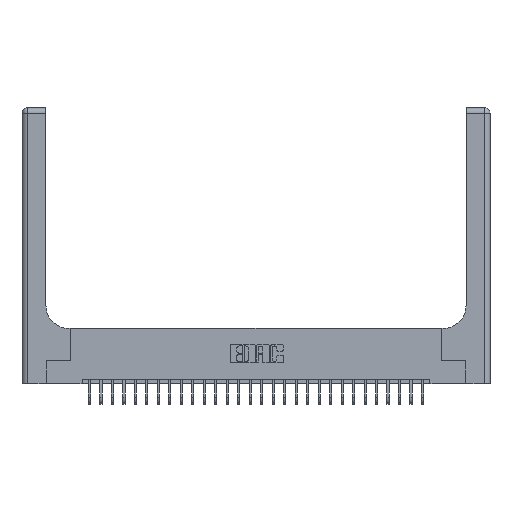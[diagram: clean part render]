
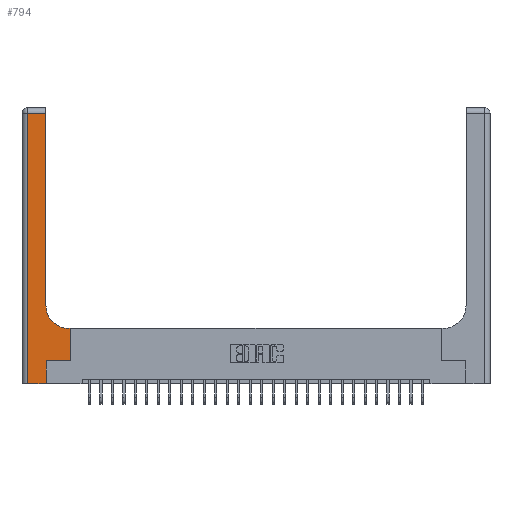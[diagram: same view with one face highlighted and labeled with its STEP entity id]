
A CAD part, top view. The second image highlights one B-rep face of the part: STEP entity #794.
In plain terms, the highlighted planar face has unit normal (0, 0, 1).
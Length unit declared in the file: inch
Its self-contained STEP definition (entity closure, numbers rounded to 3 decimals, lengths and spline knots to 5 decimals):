
#527 = VERTEX_POINT ( 'NONE', #1712 ) ;
#631 = CARTESIAN_POINT ( 'NONE',  ( 0., 2.94, 0.37 ) ) ;
#794 = ADVANCED_FACE ( 'NONE', ( #4896 ), #15321, .F. ) ;
#1518 = ORIENTED_EDGE ( 'NONE', *, *, #18836, .T. ) ;
#1706 = CARTESIAN_POINT ( 'NONE',  ( 0.265, 0.25, 0.37 ) ) ;
#1712 = CARTESIAN_POINT ( 'NONE',  ( 0.528, 0.25, 0.37 ) ) ;
#1751 = CARTESIAN_POINT ( 'NONE',  ( 0.26, 2.94, 0.37 ) ) ;
#1921 = LINE ( 'NONE', #13570, #9097 ) ;
#2032 = ORIENTED_EDGE ( 'NONE', *, *, #19525, .T. ) ;
#2452 = EDGE_CURVE ( 'NONE', #12728, #11250, #26601, .T. ) ;
#3324 = EDGE_CURVE ( 'NONE', #16595, #26419, #27912, .T. ) ;
#3382 = DIRECTION ( 'NONE',  ( 0., 1., 0. ) ) ;
#4296 = DIRECTION ( 'NONE',  ( -1., 0., 0. ) ) ;
#4558 = CARTESIAN_POINT ( 'NONE',  ( 0.06, 2.94, 0.37 ) ) ;
#4566 = CIRCLE ( 'NONE', #7201, 0.25 ) ;
#4896 = FACE_OUTER_BOUND ( 'NONE', #13126, .T. ) ;
#5246 = LINE ( 'NONE', #7978, #27718 ) ;
#5678 = CARTESIAN_POINT ( 'NONE',  ( 0.265, 0., 0.37 ) ) ;
#6216 = CARTESIAN_POINT ( 'NONE',  ( 0.06, 3., 0.37 ) ) ;
#6249 = VECTOR ( 'NONE', #9983, 39.37008 ) ;
#6709 = VERTEX_POINT ( 'NONE', #11661 ) ;
#6754 = VERTEX_POINT ( 'NONE', #14479 ) ;
#7201 = AXIS2_PLACEMENT_3D ( 'NONE', #7893, #12264, #7983 ) ;
#7348 = VECTOR ( 'NONE', #16913, 39.37008 ) ;
#7893 = CARTESIAN_POINT ( 'NONE',  ( 0.51, 0.85, 0.37 ) ) ;
#7978 = CARTESIAN_POINT ( 'NONE',  ( 0.26, 3., 0.37 ) ) ;
#7983 = DIRECTION ( 'NONE',  ( 1., 0., 0. ) ) ;
#8433 = DIRECTION ( 'NONE',  ( 1., 0., 0. ) ) ;
#8619 = CARTESIAN_POINT ( 'NONE',  ( 0., 0., 0.37 ) ) ;
#8766 = CARTESIAN_POINT ( 'NONE',  ( 0., 3., 0.37 ) ) ;
#9097 = VECTOR ( 'NONE', #9546, 39.37008 ) ;
#9546 = DIRECTION ( 'NONE',  ( 0., 1., 0. ) ) ;
#9580 = ORIENTED_EDGE ( 'NONE', *, *, #12456, .T. ) ;
#9902 = ORIENTED_EDGE ( 'NONE', *, *, #3324, .T. ) ;
#9909 = CARTESIAN_POINT ( 'NONE',  ( 0.26, 0.6, 0.37 ) ) ;
#9983 = DIRECTION ( 'NONE',  ( 0., 1., 0. ) ) ;
#10342 = LINE ( 'NONE', #20713, #6249 ) ;
#10442 = EDGE_CURVE ( 'NONE', #22441, #527, #16420, .T. ) ;
#11250 = VERTEX_POINT ( 'NONE', #4558 ) ;
#11661 = CARTESIAN_POINT ( 'NONE',  ( 0.51, 0.6, 0.37 ) ) ;
#12264 = DIRECTION ( 'NONE',  ( 0., 0., -1. ) ) ;
#12456 = EDGE_CURVE ( 'NONE', #11250, #16595, #25415, .T. ) ;
#12728 = VERTEX_POINT ( 'NONE', #1751 ) ;
#13126 = EDGE_LOOP ( 'NONE', ( #2032, #13811, #9580, #9902, #1518, #13508, #14850, #14768, #16028 ) ) ;
#13508 = ORIENTED_EDGE ( 'NONE', *, *, #10442, .T. ) ;
#13570 = CARTESIAN_POINT ( 'NONE',  ( 0.265, 0., 0.37 ) ) ;
#13811 = ORIENTED_EDGE ( 'NONE', *, *, #2452, .T. ) ;
#14378 = EDGE_CURVE ( 'NONE', #527, #17752, #10342, .T. ) ;
#14479 = CARTESIAN_POINT ( 'NONE',  ( 0.26, 0.85, 0.37 ) ) ;
#14768 = ORIENTED_EDGE ( 'NONE', *, *, #17083, .T. ) ;
#14850 = ORIENTED_EDGE ( 'NONE', *, *, #14378, .T. ) ;
#15321 = PLANE ( 'NONE',  #19387 ) ;
#15570 = CARTESIAN_POINT ( 'NONE',  ( 0.06, 0., 0.37 ) ) ;
#15729 = CARTESIAN_POINT ( 'NONE',  ( 0.528, 0.6, 0.37 ) ) ;
#16028 = ORIENTED_EDGE ( 'NONE', *, *, #20283, .T. ) ;
#16420 = LINE ( 'NONE', #1706, #17117 ) ;
#16595 = VERTEX_POINT ( 'NONE', #15570 ) ;
#16596 = VECTOR ( 'NONE', #4296, 39.37008 ) ;
#16913 = DIRECTION ( 'NONE',  ( 0., -1., 0. ) ) ;
#17083 = EDGE_CURVE ( 'NONE', #17752, #6709, #25807, .T. ) ;
#17117 = VECTOR ( 'NONE', #27949, 39.37008 ) ;
#17752 = VERTEX_POINT ( 'NONE', #15729 ) ;
#18836 = EDGE_CURVE ( 'NONE', #26419, #22441, #1921, .T. ) ;
#19387 = AXIS2_PLACEMENT_3D ( 'NONE', #8766, #28134, #24049 ) ;
#19525 = EDGE_CURVE ( 'NONE', #6754, #12728, #5246, .T. ) ;
#20143 = VECTOR ( 'NONE', #24590, 39.37008 ) ;
#20185 = CARTESIAN_POINT ( 'NONE',  ( 0.265, 0.25, 0.37 ) ) ;
#20283 = EDGE_CURVE ( 'NONE', #6709, #6754, #4566, .T. ) ;
#20713 = CARTESIAN_POINT ( 'NONE',  ( 0.528, 0.25, 0.37 ) ) ;
#22113 = VECTOR ( 'NONE', #8433, 39.37008 ) ;
#22441 = VERTEX_POINT ( 'NONE', #20185 ) ;
#24049 = DIRECTION ( 'NONE',  ( -1., 0., 0. ) ) ;
#24590 = DIRECTION ( 'NONE',  ( -1., 0., 0. ) ) ;
#25415 = LINE ( 'NONE', #6216, #7348 ) ;
#25807 = LINE ( 'NONE', #9909, #16596 ) ;
#26419 = VERTEX_POINT ( 'NONE', #5678 ) ;
#26601 = LINE ( 'NONE', #631, #20143 ) ;
#27718 = VECTOR ( 'NONE', #3382, 39.37008 ) ;
#27912 = LINE ( 'NONE', #8619, #22113 ) ;
#27949 = DIRECTION ( 'NONE',  ( 1., 0., 0. ) ) ;
#28134 = DIRECTION ( 'NONE',  ( 0., 0., -1. ) ) ;
